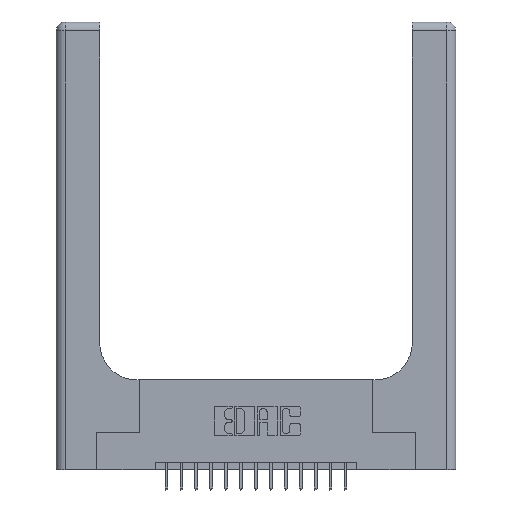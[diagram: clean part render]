
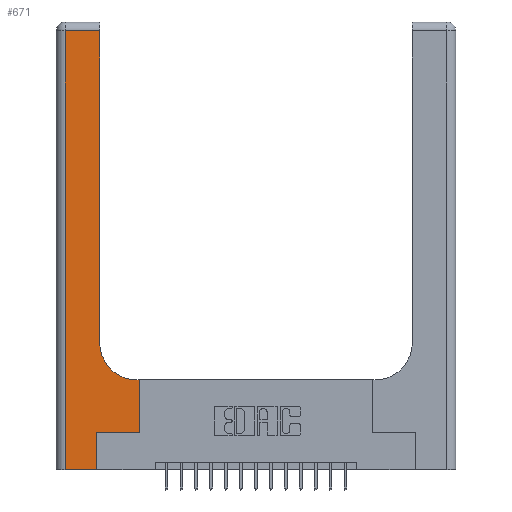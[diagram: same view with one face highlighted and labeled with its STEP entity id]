
A CAD part, top view. The second image highlights one B-rep face of the part: STEP entity #671.
In plain terms, the highlighted planar face has unit normal (0, 0, 1).
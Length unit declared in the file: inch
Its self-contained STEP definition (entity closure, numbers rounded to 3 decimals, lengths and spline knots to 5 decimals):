
#47 = CARTESIAN_POINT ( 'NONE',  ( 0.5585, 0.25, 0.37 ) ) ;
#268 = VECTOR ( 'NONE', #16701, 39.37008 ) ;
#494 = DIRECTION ( 'NONE',  ( -1., 0., 0. ) ) ;
#655 = ORIENTED_EDGE ( 'NONE', *, *, #4890, .T. ) ;
#671 = ADVANCED_FACE ( 'NONE', ( #2059 ), #15033, .F. ) ;
#898 = CARTESIAN_POINT ( 'NONE',  ( 0.5585, 0.25, 0.37 ) ) ;
#1104 = CARTESIAN_POINT ( 'NONE',  ( 0.269, 0.25, 0.37 ) ) ;
#1150 = CARTESIAN_POINT ( 'NONE',  ( 0.5415, 0.6, 0.37 ) ) ;
#1445 = EDGE_CURVE ( 'NONE', #11252, #13131, #10176, .T. ) ;
#1705 = CARTESIAN_POINT ( 'NONE',  ( 0.269, 0.25, 0.37 ) ) ;
#2059 = FACE_OUTER_BOUND ( 'NONE', #11613, .T. ) ;
#3441 = ORIENTED_EDGE ( 'NONE', *, *, #16670, .T. ) ;
#3973 = VECTOR ( 'NONE', #4715, 39.37008 ) ;
#4165 = ORIENTED_EDGE ( 'NONE', *, *, #17745, .T. ) ;
#4559 = ORIENTED_EDGE ( 'NONE', *, *, #6690, .T. ) ;
#4623 = EDGE_CURVE ( 'NONE', #6523, #8854, #9066, .T. ) ;
#4715 = DIRECTION ( 'NONE',  ( -1., 0., 0. ) ) ;
#4790 = VERTEX_POINT ( 'NONE', #16924 ) ;
#4890 = EDGE_CURVE ( 'NONE', #10838, #4790, #12886, .T. ) ;
#5533 = CARTESIAN_POINT ( 'NONE',  ( 0.5585, 0.6, 0.37 ) ) ;
#6004 = DIRECTION ( 'NONE',  ( 0., -1., 0. ) ) ;
#6180 = LINE ( 'NONE', #11089, #3973 ) ;
#6414 = EDGE_CURVE ( 'NONE', #13131, #6523, #9071, .T. ) ;
#6523 = VERTEX_POINT ( 'NONE', #898 ) ;
#6690 = EDGE_CURVE ( 'NONE', #12201, #10838, #19133, .T. ) ;
#6727 = EDGE_CURVE ( 'NONE', #4790, #14413, #6180, .T. ) ;
#6912 = CARTESIAN_POINT ( 'NONE',  ( 0.269, 0., 0.37 ) ) ;
#7373 = DIRECTION ( 'NONE',  ( 0., 0., -1. ) ) ;
#7472 = LINE ( 'NONE', #9240, #16733 ) ;
#7682 = AXIS2_PLACEMENT_3D ( 'NONE', #18341, #7373, #494 ) ;
#7718 = VECTOR ( 'NONE', #19281, 39.37008 ) ;
#7888 = ORIENTED_EDGE ( 'NONE', *, *, #4623, .T. ) ;
#8854 = VERTEX_POINT ( 'NONE', #5533 ) ;
#8920 = DIRECTION ( 'NONE',  ( 0., 0., -1. ) ) ;
#9066 = LINE ( 'NONE', #47, #18145 ) ;
#9071 = LINE ( 'NONE', #1705, #15211 ) ;
#9082 = VERTEX_POINT ( 'NONE', #12564 ) ;
#9135 = LINE ( 'NONE', #13540, #268 ) ;
#9240 = CARTESIAN_POINT ( 'NONE',  ( 0., 0., 0.37 ) ) ;
#9488 = ORIENTED_EDGE ( 'NONE', *, *, #6414, .T. ) ;
#10176 = LINE ( 'NONE', #16257, #7718 ) ;
#10180 = EDGE_CURVE ( 'NONE', #9082, #11252, #7472, .T. ) ;
#10646 = DIRECTION ( 'NONE',  ( 0., 1., 0. ) ) ;
#10688 = AXIS2_PLACEMENT_3D ( 'NONE', #16483, #8920, #13526 ) ;
#10838 = VERTEX_POINT ( 'NONE', #18992 ) ;
#11089 = CARTESIAN_POINT ( 'NONE',  ( 0., 2.94, 0.37 ) ) ;
#11252 = VERTEX_POINT ( 'NONE', #6912 ) ;
#11416 = DIRECTION ( 'NONE',  ( 0., 1., 0. ) ) ;
#11613 = EDGE_LOOP ( 'NONE', ( #655, #17484, #3441, #14224, #12851, #9488, #7888, #4165, #4559 ) ) ;
#12201 = VERTEX_POINT ( 'NONE', #1150 ) ;
#12384 = DIRECTION ( 'NONE',  ( 1., 0., 0. ) ) ;
#12564 = CARTESIAN_POINT ( 'NONE',  ( 0.06, 0., 0.37 ) ) ;
#12851 = ORIENTED_EDGE ( 'NONE', *, *, #1445, .T. ) ;
#12886 = LINE ( 'NONE', #18863, #16600 ) ;
#13131 = VERTEX_POINT ( 'NONE', #1104 ) ;
#13526 = DIRECTION ( 'NONE',  ( 1., 0., 0. ) ) ;
#13540 = CARTESIAN_POINT ( 'NONE',  ( 0.2915, 0.6, 0.37 ) ) ;
#14224 = ORIENTED_EDGE ( 'NONE', *, *, #10180, .T. ) ;
#14413 = VERTEX_POINT ( 'NONE', #16125 ) ;
#15010 = CARTESIAN_POINT ( 'NONE',  ( 0.06, 3., 0.37 ) ) ;
#15033 = PLANE ( 'NONE',  #7682 ) ;
#15211 = VECTOR ( 'NONE', #15511, 39.37008 ) ;
#15511 = DIRECTION ( 'NONE',  ( 1., 0., 0. ) ) ;
#16125 = CARTESIAN_POINT ( 'NONE',  ( 0.06, 2.94, 0.37 ) ) ;
#16257 = CARTESIAN_POINT ( 'NONE',  ( 0.269, 0., 0.37 ) ) ;
#16303 = LINE ( 'NONE', #15010, #18466 ) ;
#16483 = CARTESIAN_POINT ( 'NONE',  ( 0.5415, 0.85, 0.37 ) ) ;
#16600 = VECTOR ( 'NONE', #11416, 39.37008 ) ;
#16670 = EDGE_CURVE ( 'NONE', #14413, #9082, #16303, .T. ) ;
#16701 = DIRECTION ( 'NONE',  ( -1., 0., 0. ) ) ;
#16733 = VECTOR ( 'NONE', #12384, 39.37008 ) ;
#16924 = CARTESIAN_POINT ( 'NONE',  ( 0.2915, 2.94, 0.37 ) ) ;
#17484 = ORIENTED_EDGE ( 'NONE', *, *, #6727, .T. ) ;
#17745 = EDGE_CURVE ( 'NONE', #8854, #12201, #9135, .T. ) ;
#18145 = VECTOR ( 'NONE', #10646, 39.37008 ) ;
#18341 = CARTESIAN_POINT ( 'NONE',  ( 0., 3., 0.37 ) ) ;
#18466 = VECTOR ( 'NONE', #6004, 39.37008 ) ;
#18863 = CARTESIAN_POINT ( 'NONE',  ( 0.2915, 3., 0.37 ) ) ;
#18992 = CARTESIAN_POINT ( 'NONE',  ( 0.2915, 0.85, 0.37 ) ) ;
#19133 = CIRCLE ( 'NONE', #10688, 0.25 ) ;
#19281 = DIRECTION ( 'NONE',  ( 0., 1., 0. ) ) ;
